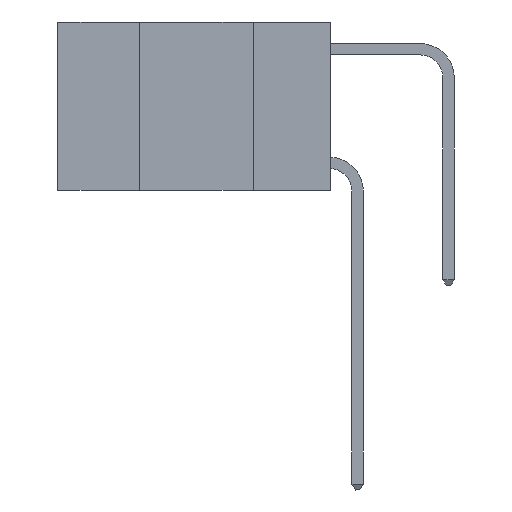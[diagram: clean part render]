
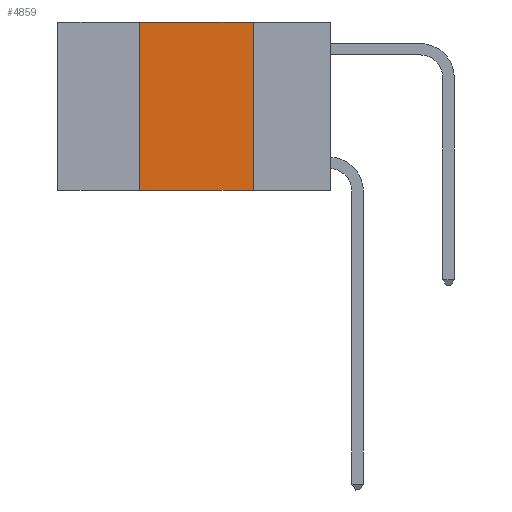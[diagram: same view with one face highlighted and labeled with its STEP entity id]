
A CAD part, left-side view. The second image highlights one B-rep face of the part: STEP entity #4859.
In plain terms, the highlighted planar face has unit normal (-1, 0, 0).
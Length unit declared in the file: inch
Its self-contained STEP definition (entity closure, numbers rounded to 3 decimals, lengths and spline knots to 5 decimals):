
#276 = EDGE_LOOP ( 'NONE', ( #13147, #800, #2352, #7636 ) ) ;
#800 = ORIENTED_EDGE ( 'NONE', *, *, #7360, .F. ) ;
#2066 = LINE ( 'NONE', #14245, #5762 ) ;
#2082 = DIRECTION ( 'NONE',  ( 0., 0., -1. ) ) ;
#2352 = ORIENTED_EDGE ( 'NONE', *, *, #8198, .F. ) ;
#2375 = LINE ( 'NONE', #11986, #11457 ) ;
#2543 = VERTEX_POINT ( 'NONE', #15199 ) ;
#2955 = VECTOR ( 'NONE', #3588, 39.37008 ) ;
#3588 = DIRECTION ( 'NONE',  ( 0., 0., -1. ) ) ;
#3932 = VERTEX_POINT ( 'NONE', #6326 ) ;
#4570 = DIRECTION ( 'NONE',  ( 0., -1., 0. ) ) ;
#4859 = ADVANCED_FACE ( 'NONE', ( #9978 ), #5672, .F. ) ;
#5013 = EDGE_CURVE ( 'NONE', #15485, #3932, #2066, .T. ) ;
#5624 = CARTESIAN_POINT ( 'NONE',  ( 0., 0.42, 0. ) ) ;
#5672 = PLANE ( 'NONE',  #12247 ) ;
#5762 = VECTOR ( 'NONE', #6849, 39.37008 ) ;
#6326 = CARTESIAN_POINT ( 'NONE',  ( 0., 0.17, -0.37 ) ) ;
#6849 = DIRECTION ( 'NONE',  ( 0., -1., 0. ) ) ;
#7360 = EDGE_CURVE ( 'NONE', #2543, #7869, #2375, .T. ) ;
#7392 = CARTESIAN_POINT ( 'NONE',  ( 0., 0.17, 0. ) ) ;
#7615 = CARTESIAN_POINT ( 'NONE',  ( 0., 0.17, 0. ) ) ;
#7636 = ORIENTED_EDGE ( 'NONE', *, *, #5013, .T. ) ;
#7869 = VERTEX_POINT ( 'NONE', #7615 ) ;
#8198 = EDGE_CURVE ( 'NONE', #15485, #2543, #12390, .T. ) ;
#9506 = VECTOR ( 'NONE', #14630, 39.37008 ) ;
#9978 = FACE_OUTER_BOUND ( 'NONE', #276, .T. ) ;
#11457 = VECTOR ( 'NONE', #4570, 39.37008 ) ;
#11986 = CARTESIAN_POINT ( 'NONE',  ( 0., 0.6, 0. ) ) ;
#12247 = AXIS2_PLACEMENT_3D ( 'NONE', #15528, #13115, #2082 ) ;
#12390 = LINE ( 'NONE', #5624, #9506 ) ;
#12965 = EDGE_CURVE ( 'NONE', #7869, #3932, #14724, .T. ) ;
#13115 = DIRECTION ( 'NONE',  ( 1., 0., 0. ) ) ;
#13147 = ORIENTED_EDGE ( 'NONE', *, *, #12965, .F. ) ;
#14245 = CARTESIAN_POINT ( 'NONE',  ( 0., 0.6, -0.37 ) ) ;
#14630 = DIRECTION ( 'NONE',  ( 0., 0., 1. ) ) ;
#14724 = LINE ( 'NONE', #7392, #2955 ) ;
#15125 = CARTESIAN_POINT ( 'NONE',  ( 0., 0.42, -0.37 ) ) ;
#15199 = CARTESIAN_POINT ( 'NONE',  ( 0., 0.42, 0. ) ) ;
#15485 = VERTEX_POINT ( 'NONE', #15125 ) ;
#15528 = CARTESIAN_POINT ( 'NONE',  ( 0., 0.6, 0. ) ) ;
